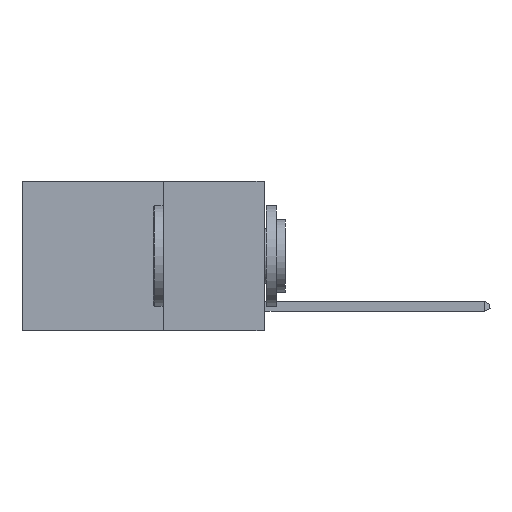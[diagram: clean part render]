
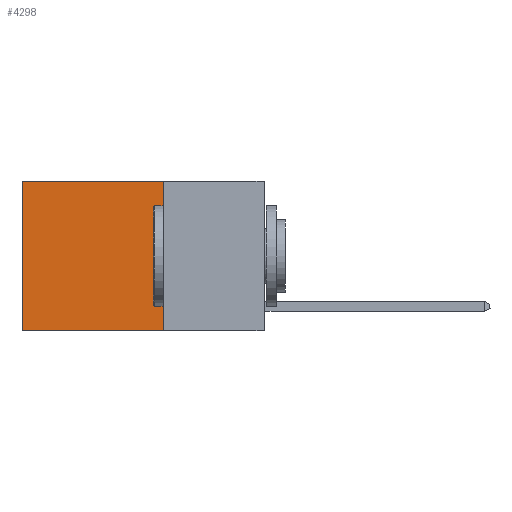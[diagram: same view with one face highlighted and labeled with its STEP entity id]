
A CAD part, left-side view. The second image highlights one B-rep face of the part: STEP entity #4298.
In plain terms, the highlighted planar face has unit normal (-1, 0, 0).
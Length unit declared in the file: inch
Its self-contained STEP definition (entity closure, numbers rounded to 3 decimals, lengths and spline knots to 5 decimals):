
#35 = VERTEX_POINT ( 'NONE', #7512 ) ;
#531 = CARTESIAN_POINT ( 'NONE',  ( 0.2625, 0.6, 0. ) ) ;
#573 = VECTOR ( 'NONE', #9511, 39.37008 ) ;
#1018 = AXIS2_PLACEMENT_3D ( 'NONE', #8598, #4884, #8515 ) ;
#1129 = DIRECTION ( 'NONE',  ( 0., 0., -1. ) ) ;
#1397 = CARTESIAN_POINT ( 'NONE',  ( 0.2625, 0.6, 0. ) ) ;
#1586 = DIRECTION ( 'NONE',  ( 0., 1., 0. ) ) ;
#1812 = EDGE_CURVE ( 'NONE', #6453, #35, #9055, .T. ) ;
#2533 = ORIENTED_EDGE ( 'NONE', *, *, #11860, .T. ) ;
#3001 = ORIENTED_EDGE ( 'NONE', *, *, #1812, .F. ) ;
#4298 = ADVANCED_FACE ( 'NONE', ( #16262 ), #9923, .F. ) ;
#4884 = DIRECTION ( 'NONE',  ( 1., 0., 0. ) ) ;
#5507 = VERTEX_POINT ( 'NONE', #6123 ) ;
#5894 = VECTOR ( 'NONE', #1129, 39.37008 ) ;
#6123 = CARTESIAN_POINT ( 'NONE',  ( 0.2625, 0.25, 0. ) ) ;
#6431 = CARTESIAN_POINT ( 'NONE',  ( 0.2625, 0.25, -0.37 ) ) ;
#6453 = VERTEX_POINT ( 'NONE', #9151 ) ;
#7006 = ORIENTED_EDGE ( 'NONE', *, *, #11489, .F. ) ;
#7512 = CARTESIAN_POINT ( 'NONE',  ( 0.2625, 0.6, -0.37 ) ) ;
#8440 = VECTOR ( 'NONE', #1586, 39.37008 ) ;
#8515 = DIRECTION ( 'NONE',  ( 0., 0., -1. ) ) ;
#8529 = CARTESIAN_POINT ( 'NONE',  ( 0.2625, 0.25, 0. ) ) ;
#8598 = CARTESIAN_POINT ( 'NONE',  ( 0.2625, 0.25, 0. ) ) ;
#8959 = CARTESIAN_POINT ( 'NONE',  ( 0.2625, 0.25, 0. ) ) ;
#9055 = LINE ( 'NONE', #6431, #8440 ) ;
#9151 = CARTESIAN_POINT ( 'NONE',  ( 0.2625, 0.25, -0.37 ) ) ;
#9393 = EDGE_LOOP ( 'NONE', ( #2533, #3001, #7006, #13018 ) ) ;
#9511 = DIRECTION ( 'NONE',  ( 0., 0., -1. ) ) ;
#9923 = PLANE ( 'NONE',  #1018 ) ;
#11489 = EDGE_CURVE ( 'NONE', #5507, #6453, #14948, .T. ) ;
#11794 = LINE ( 'NONE', #8959, #12029 ) ;
#11860 = EDGE_CURVE ( 'NONE', #12636, #35, #11931, .T. ) ;
#11931 = LINE ( 'NONE', #531, #573 ) ;
#12029 = VECTOR ( 'NONE', #15636, 39.37008 ) ;
#12571 = EDGE_CURVE ( 'NONE', #5507, #12636, #11794, .T. ) ;
#12636 = VERTEX_POINT ( 'NONE', #1397 ) ;
#13018 = ORIENTED_EDGE ( 'NONE', *, *, #12571, .T. ) ;
#14948 = LINE ( 'NONE', #8529, #5894 ) ;
#15636 = DIRECTION ( 'NONE',  ( 0., 1., 0. ) ) ;
#16262 = FACE_OUTER_BOUND ( 'NONE', #9393, .T. ) ;
